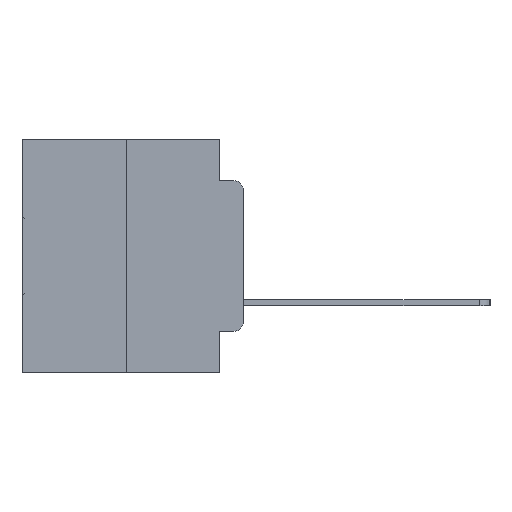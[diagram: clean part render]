
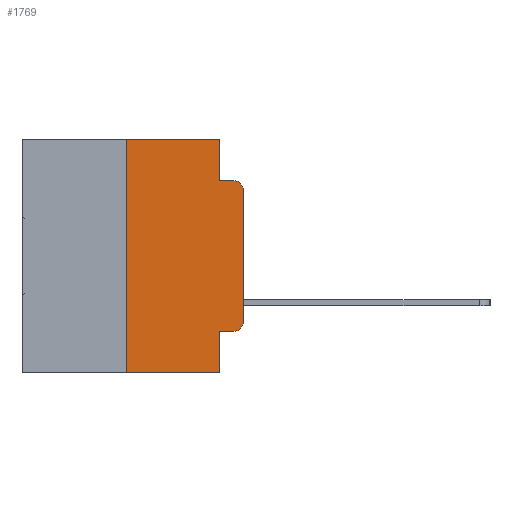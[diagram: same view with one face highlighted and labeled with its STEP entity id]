
A CAD part, left-side view. The second image highlights one B-rep face of the part: STEP entity #1769.
In plain terms, the highlighted planar face has unit normal (-1, 0, 0).
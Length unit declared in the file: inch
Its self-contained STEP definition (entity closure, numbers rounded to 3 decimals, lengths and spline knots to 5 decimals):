
#103 = VECTOR ( 'NONE', #18992, 39.37008 ) ;
#371 = CARTESIAN_POINT ( 'NONE',  ( 0., 0.02, -0.3915 ) ) ;
#590 = DIRECTION ( 'NONE',  ( 0., -1., 0. ) ) ;
#784 = VECTOR ( 'NONE', #29599, 39.37008 ) ;
#846 = EDGE_CURVE ( 'NONE', #19711, #18238, #18274, .T. ) ;
#1413 = AXIS2_PLACEMENT_3D ( 'NONE', #14481, #14239, #13045 ) ;
#1443 = DIRECTION ( 'NONE',  ( 0., 0., -1. ) ) ;
#1618 = DIRECTION ( 'NONE',  ( 1., 0., 0. ) ) ;
#1769 = ADVANCED_FACE ( 'NONE', ( #24665 ), #28476, .F. ) ;
#2110 = LINE ( 'NONE', #26916, #13602 ) ;
#2378 = ORIENTED_EDGE ( 'NONE', *, *, #25104, .F. ) ;
#2844 = DIRECTION ( 'NONE',  ( 0., 0., -1. ) ) ;
#3535 = EDGE_CURVE ( 'NONE', #17683, #8834, #13806, .T. ) ;
#3929 = ORIENTED_EDGE ( 'NONE', *, *, #21411, .T. ) ;
#4218 = VECTOR ( 'NONE', #22053, 39.37008 ) ;
#5093 = ORIENTED_EDGE ( 'NONE', *, *, #12342, .F. ) ;
#5228 = CARTESIAN_POINT ( 'NONE',  ( 0., 0.473, -0.5 ) ) ;
#5826 = LINE ( 'NONE', #16204, #30411 ) ;
#6531 = VERTEX_POINT ( 'NONE', #18488 ) ;
#7055 = VERTEX_POINT ( 'NONE', #10806 ) ;
#7465 = LINE ( 'NONE', #9502, #103 ) ;
#8533 = EDGE_CURVE ( 'NONE', #17683, #17497, #7465, .T. ) ;
#8834 = VERTEX_POINT ( 'NONE', #10713 ) ;
#9083 = LINE ( 'NONE', #15237, #27322 ) ;
#9333 = ORIENTED_EDGE ( 'NONE', *, *, #846, .T. ) ;
#9393 = CARTESIAN_POINT ( 'NONE',  ( 0., 0.02, -0.4115 ) ) ;
#9502 = CARTESIAN_POINT ( 'NONE',  ( 0., 0.051, -0.4115 ) ) ;
#9977 = LINE ( 'NONE', #5228, #4218 ) ;
#10622 = CARTESIAN_POINT ( 'NONE',  ( 0., 0.051, 0. ) ) ;
#10713 = CARTESIAN_POINT ( 'NONE',  ( 0., 0.051, -0.5 ) ) ;
#10806 = CARTESIAN_POINT ( 'NONE',  ( 0., 0.25, 0. ) ) ;
#10966 = LINE ( 'NONE', #11879, #23664 ) ;
#11357 = CARTESIAN_POINT ( 'NONE',  ( 0., 0., -0.3915 ) ) ;
#11879 = CARTESIAN_POINT ( 'NONE',  ( 0., 0.051, -0.0885 ) ) ;
#12342 = EDGE_CURVE ( 'NONE', #17527, #18238, #10966, .T. ) ;
#12597 = EDGE_CURVE ( 'NONE', #7055, #30550, #9083, .T. ) ;
#13045 = DIRECTION ( 'NONE',  ( 0., 0., -1. ) ) ;
#13602 = VECTOR ( 'NONE', #29240, 39.37008 ) ;
#13806 = LINE ( 'NONE', #10622, #784 ) ;
#14239 = DIRECTION ( 'NONE',  ( -1., 0., 0. ) ) ;
#14481 = CARTESIAN_POINT ( 'NONE',  ( 0., 0.02, -0.1085 ) ) ;
#15237 = CARTESIAN_POINT ( 'NONE',  ( 0., 0.473, 0. ) ) ;
#16204 = CARTESIAN_POINT ( 'NONE',  ( 0., 0.051, 0. ) ) ;
#16598 = EDGE_CURVE ( 'NONE', #17497, #20494, #19526, .T. ) ;
#17397 = DIRECTION ( 'NONE',  ( -1., 0., 0. ) ) ;
#17497 = VERTEX_POINT ( 'NONE', #9393 ) ;
#17527 = VERTEX_POINT ( 'NONE', #26051 ) ;
#17587 = CARTESIAN_POINT ( 'NONE',  ( 0., 0.473, 0. ) ) ;
#17683 = VERTEX_POINT ( 'NONE', #22011 ) ;
#18238 = VERTEX_POINT ( 'NONE', #19094 ) ;
#18274 = CIRCLE ( 'NONE', #1413, 0.02 ) ;
#18488 = CARTESIAN_POINT ( 'NONE',  ( 0., 0.25, -0.5 ) ) ;
#18757 = EDGE_CURVE ( 'NONE', #30550, #17527, #5826, .T. ) ;
#18992 = DIRECTION ( 'NONE',  ( 0., -1., 0. ) ) ;
#19066 = ORIENTED_EDGE ( 'NONE', *, *, #8533, .T. ) ;
#19094 = CARTESIAN_POINT ( 'NONE',  ( 0., 0.02, -0.0885 ) ) ;
#19271 = CARTESIAN_POINT ( 'NONE',  ( 0., 0.25, 0. ) ) ;
#19526 = CIRCLE ( 'NONE', #22402, 0.02 ) ;
#19711 = VERTEX_POINT ( 'NONE', #20369 ) ;
#20369 = CARTESIAN_POINT ( 'NONE',  ( 0., 0., -0.1085 ) ) ;
#20494 = VERTEX_POINT ( 'NONE', #11357 ) ;
#20563 = ORIENTED_EDGE ( 'NONE', *, *, #16598, .T. ) ;
#20921 = ORIENTED_EDGE ( 'NONE', *, *, #12597, .F. ) ;
#21411 = EDGE_CURVE ( 'NONE', #6531, #8834, #9977, .T. ) ;
#21677 = DIRECTION ( 'NONE',  ( 0., 0., 1. ) ) ;
#22011 = CARTESIAN_POINT ( 'NONE',  ( 0., 0.051, -0.4115 ) ) ;
#22053 = DIRECTION ( 'NONE',  ( 0., -1., 0. ) ) ;
#22402 = AXIS2_PLACEMENT_3D ( 'NONE', #371, #17397, #2844 ) ;
#22783 = VECTOR ( 'NONE', #21677, 39.37008 ) ;
#23550 = LINE ( 'NONE', #19271, #22783 ) ;
#23664 = VECTOR ( 'NONE', #28478, 39.37008 ) ;
#23896 = AXIS2_PLACEMENT_3D ( 'NONE', #17587, #1618, #1443 ) ;
#23905 = ORIENTED_EDGE ( 'NONE', *, *, #3535, .F. ) ;
#24665 = FACE_OUTER_BOUND ( 'NONE', #25396, .T. ) ;
#25104 = EDGE_CURVE ( 'NONE', #6531, #7055, #23550, .T. ) ;
#25396 = EDGE_LOOP ( 'NONE', ( #26833, #9333, #5093, #25725, #20921, #2378, #3929, #23905, #19066, #20563 ) ) ;
#25725 = ORIENTED_EDGE ( 'NONE', *, *, #18757, .F. ) ;
#26051 = CARTESIAN_POINT ( 'NONE',  ( 0., 0.051, -0.0885 ) ) ;
#26833 = ORIENTED_EDGE ( 'NONE', *, *, #27282, .T. ) ;
#26916 = CARTESIAN_POINT ( 'NONE',  ( 0., 0., 0. ) ) ;
#27009 = CARTESIAN_POINT ( 'NONE',  ( 0., 0.051, 0. ) ) ;
#27282 = EDGE_CURVE ( 'NONE', #20494, #19711, #2110, .T. ) ;
#27322 = VECTOR ( 'NONE', #590, 39.37008 ) ;
#28476 = PLANE ( 'NONE',  #23896 ) ;
#28478 = DIRECTION ( 'NONE',  ( 0., -1., 0. ) ) ;
#29240 = DIRECTION ( 'NONE',  ( 0., 0., 1. ) ) ;
#29599 = DIRECTION ( 'NONE',  ( 0., 0., -1. ) ) ;
#30383 = DIRECTION ( 'NONE',  ( 0., 0., -1. ) ) ;
#30411 = VECTOR ( 'NONE', #30383, 39.37008 ) ;
#30550 = VERTEX_POINT ( 'NONE', #27009 ) ;
